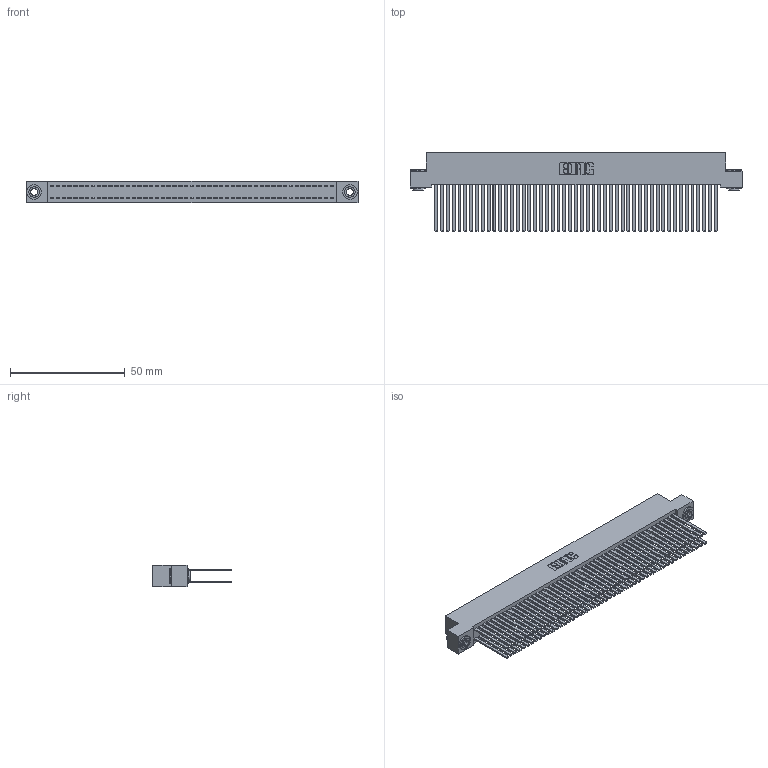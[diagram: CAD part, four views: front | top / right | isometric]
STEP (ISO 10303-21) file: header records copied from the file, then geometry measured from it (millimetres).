
FILE_DESCRIPTION (( 'STEP AP203' ), '1' );
FILE_NAME ('392-098-544-203.STEP', '2019-10-09T20:26:48', ( '' ), ( '' ), 'SwSTEP 2.0', 'SolidWorks 2016', '' );
FILE_SCHEMA (( 'CONFIG_CONTROL_DESIGN' ));
Length unit declared in the file: inch
Products named in the file (4): 342 Part_.156 TH; 345-292-001_345-293-144; 342-250-002_345-250-002-102; 392-098-544-203
Assembly tree (101 placements, depth 2):
  392-098-544-203
    342 Part_.156 TH
    345-292-001_345-293-144  x98
    342-250-002_345-250-002-102  x2
Bounding box: 144.78 x 34.3 x 9.4 mm (x, y, z)
Volume: 14438.2 mm3; surface area: 27692.8 mm2
Topology: 101 solids, 101 shells, 4656 faces, 13801 edges, 9066 vertices
Faces by surface type: plane 3212, cylinder 1436, cone 8
Entity records: 30952 total; most frequent: CARTESIAN_POINT 5093, ORIENTED_EDGE 5022, DIRECTION 4369, EDGE_CURVE 2511, VECTOR 2363, LINE 2363, VERTEX_POINT 1670, AXIS2_PLACEMENT_3D 1003
